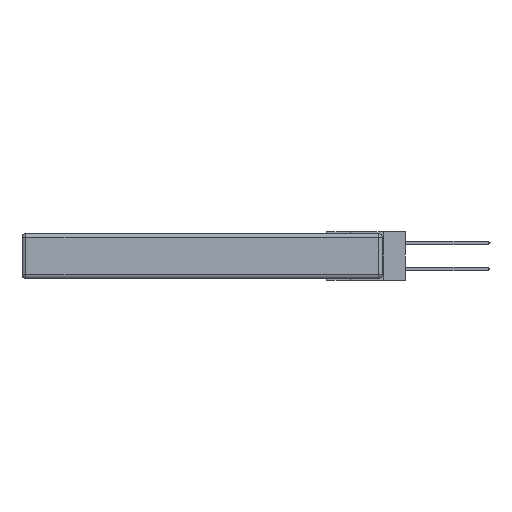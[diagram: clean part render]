
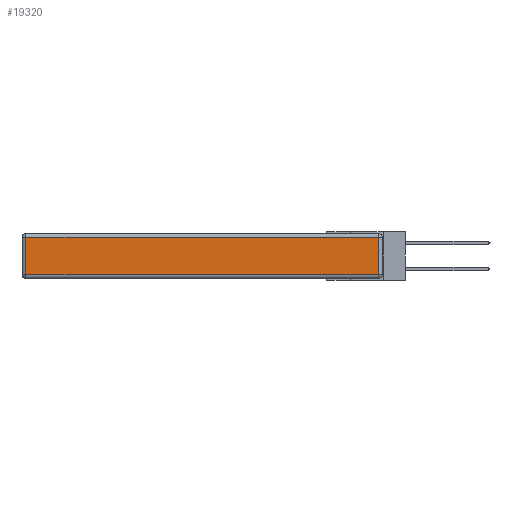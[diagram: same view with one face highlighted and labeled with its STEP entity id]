
A CAD part, left-side view. The second image highlights one B-rep face of the part: STEP entity #19320.
In plain terms, the highlighted planar face has unit normal (-1, 0, 0).
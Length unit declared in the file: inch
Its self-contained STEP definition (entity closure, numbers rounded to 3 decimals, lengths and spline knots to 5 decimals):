
#1457 = EDGE_CURVE ( 'NONE', #1608, #18577, #14884, .T. ) ;
#1608 = VERTEX_POINT ( 'NONE', #12896 ) ;
#1872 = DIRECTION ( 'NONE',  ( -1., 0., 0. ) ) ;
#2678 = AXIS2_PLACEMENT_3D ( 'NONE', #19753, #1872, #18181 ) ;
#2812 = DIRECTION ( 'NONE',  ( 0., -1., 0. ) ) ;
#3410 = FACE_OUTER_BOUND ( 'NONE', #21559, .T. ) ;
#4977 = VERTEX_POINT ( 'NONE', #22728 ) ;
#6508 = VECTOR ( 'NONE', #2812, 39.37008 ) ;
#7054 = LINE ( 'NONE', #22285, #6508 ) ;
#8158 = DIRECTION ( 'NONE',  ( 0., 1., 0. ) ) ;
#8807 = VERTEX_POINT ( 'NONE', #14999 ) ;
#10046 = LINE ( 'NONE', #18314, #21866 ) ;
#10281 = ORIENTED_EDGE ( 'NONE', *, *, #1457, .T. ) ;
#11220 = EDGE_CURVE ( 'NONE', #8807, #4977, #10046, .T. ) ;
#12896 = CARTESIAN_POINT ( 'NONE',  ( 0., 0.03, -0.313 ) ) ;
#13512 = CARTESIAN_POINT ( 'NONE',  ( 0., 2.75, -0.03 ) ) ;
#14782 = ORIENTED_EDGE ( 'NONE', *, *, #19703, .T. ) ;
#14884 = LINE ( 'NONE', #15916, #17709 ) ;
#14999 = CARTESIAN_POINT ( 'NONE',  ( 0., 2.72, -0.03 ) ) ;
#15037 = DIRECTION ( 'NONE',  ( 0., 0., -1. ) ) ;
#15701 = ORIENTED_EDGE ( 'NONE', *, *, #16232, .T. ) ;
#15718 = CARTESIAN_POINT ( 'NONE',  ( 0., 0.03, -0.03 ) ) ;
#15916 = CARTESIAN_POINT ( 'NONE',  ( 0., 0.03, -0.343 ) ) ;
#16232 = EDGE_CURVE ( 'NONE', #18577, #8807, #20119, .T. ) ;
#17709 = VECTOR ( 'NONE', #21078, 39.37008 ) ;
#17729 = PLANE ( 'NONE',  #2678 ) ;
#18181 = DIRECTION ( 'NONE',  ( 0., 0., 1. ) ) ;
#18314 = CARTESIAN_POINT ( 'NONE',  ( 0., 2.72, -0.343 ) ) ;
#18577 = VERTEX_POINT ( 'NONE', #15718 ) ;
#19177 = ORIENTED_EDGE ( 'NONE', *, *, #11220, .T. ) ;
#19320 = ADVANCED_FACE ( 'NONE', ( #3410 ), #17729, .T. ) ;
#19703 = EDGE_CURVE ( 'NONE', #4977, #1608, #7054, .T. ) ;
#19753 = CARTESIAN_POINT ( 'NONE',  ( 0., 0., -0.343 ) ) ;
#20119 = LINE ( 'NONE', #13512, #21247 ) ;
#21078 = DIRECTION ( 'NONE',  ( 0., 0., 1. ) ) ;
#21247 = VECTOR ( 'NONE', #8158, 39.37008 ) ;
#21559 = EDGE_LOOP ( 'NONE', ( #14782, #10281, #15701, #19177 ) ) ;
#21866 = VECTOR ( 'NONE', #15037, 39.37008 ) ;
#22285 = CARTESIAN_POINT ( 'NONE',  ( 0., 0., -0.313 ) ) ;
#22728 = CARTESIAN_POINT ( 'NONE',  ( 0., 2.72, -0.313 ) ) ;
